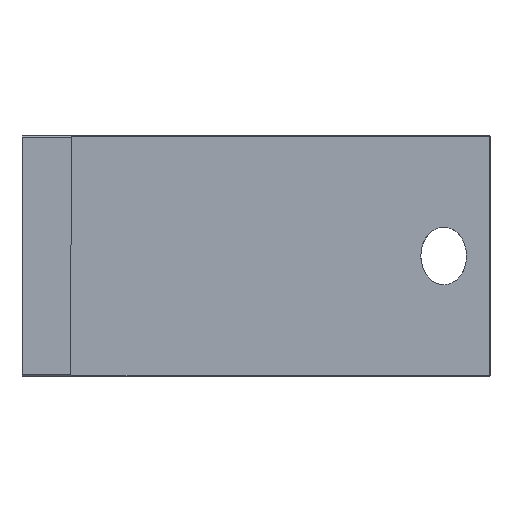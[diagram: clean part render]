
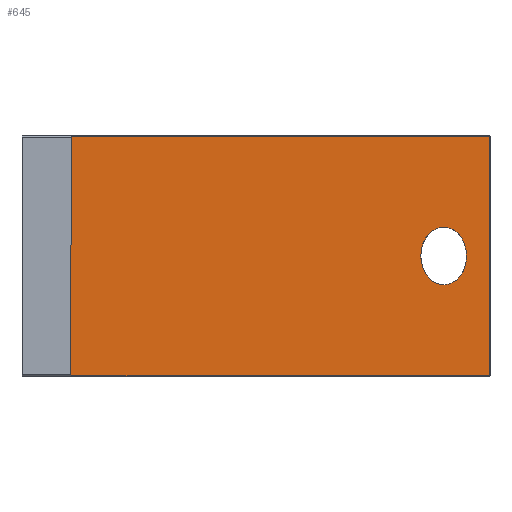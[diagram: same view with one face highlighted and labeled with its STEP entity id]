
A CAD part, left-side view. The second image highlights one B-rep face of the part: STEP entity #645.
In plain terms, the highlighted planar face has unit normal (-1, 0, 0).
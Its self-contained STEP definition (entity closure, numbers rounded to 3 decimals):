
#16=FACE_BOUND('',#121,.T.);
#17=ELLIPSE('',#684,1.104,0.873);
#18=ELLIPSE('',#685,1.104,0.873);
#49=PLANE('',#711);
#84=FACE_OUTER_BOUND('',#120,.T.);
#120=EDGE_LOOP('',(#591,#592,#593,#594));
#121=EDGE_LOOP('',(#595,#596));
#178=LINE('',#1037,#255);
#191=LINE('',#1061,#268);
#194=LINE('',#1067,#271);
#199=LINE('',#1078,#276);
#255=VECTOR('',#830,10.);
#268=VECTOR('',#855,10.);
#271=VECTOR('',#862,10.);
#276=VECTOR('',#877,1000.);
#310=VERTEX_POINT('',#967);
#311=VERTEX_POINT('',#968);
#332=VERTEX_POINT('',#1029);
#334=VERTEX_POINT('',#1035);
#338=VERTEX_POINT('',#1054);
#340=VERTEX_POINT('',#1065);
#373=EDGE_CURVE('',#310,#311,#17,.T.);
#374=EDGE_CURVE('',#311,#310,#18,.T.);
#408=EDGE_CURVE('',#332,#334,#178,.T.);
#421=EDGE_CURVE('',#338,#332,#191,.T.);
#424=EDGE_CURVE('',#340,#338,#194,.T.);
#429=EDGE_CURVE('',#340,#334,#199,.T.);
#591=ORIENTED_EDGE('',*,*,#424,.F.);
#592=ORIENTED_EDGE('',*,*,#429,.T.);
#593=ORIENTED_EDGE('',*,*,#408,.F.);
#594=ORIENTED_EDGE('',*,*,#421,.F.);
#595=ORIENTED_EDGE('',*,*,#373,.T.);
#596=ORIENTED_EDGE('',*,*,#374,.T.);
#645=ADVANCED_FACE('',(#84,#16),#49,.F.);
#684=AXIS2_PLACEMENT_3D('',#969,#771,#772);
#685=AXIS2_PLACEMENT_3D('',#970,#773,#774);
#711=AXIS2_PLACEMENT_3D('',#1079,#878,#879);
#771=DIRECTION('center_axis',(1.,0.,0.));
#772=DIRECTION('ref_axis',(0.,0.,1.));
#773=DIRECTION('center_axis',(1.,0.,0.));
#774=DIRECTION('ref_axis',(0.,0.,1.));
#830=DIRECTION('',(0.,1.,0.));
#855=DIRECTION('',(0.,0.,-1.));
#862=DIRECTION('',(0.,-1.,0.));
#877=DIRECTION('',(0.,0.001,-1.));
#878=DIRECTION('center_axis',(1.,0.,0.));
#879=DIRECTION('ref_axis',(0.,1.,0.));
#967=CARTESIAN_POINT('',(-14.424,-19.812,5.704));
#968=CARTESIAN_POINT('',(-14.424,-19.812,3.496));
#969=CARTESIAN_POINT('Origin',(-14.424,-19.812,4.6));
#970=CARTESIAN_POINT('Origin',(-14.424,-19.812,4.6));
#1029=CARTESIAN_POINT('',(-14.424,-21.577,0.01));
#1035=CARTESIAN_POINT('',(-14.424,-5.53,0.01));
#1037=CARTESIAN_POINT('',(-14.424,-10.794,0.01));
#1054=CARTESIAN_POINT('',(-14.424,-21.577,9.19));
#1061=CARTESIAN_POINT('',(-14.424,-21.577,9.2));
#1065=CARTESIAN_POINT('',(-14.424,-5.538,9.19));
#1067=CARTESIAN_POINT('',(-14.424,-10.794,9.19));
#1078=CARTESIAN_POINT('',(-14.424,-5.538,9.2));
#1079=CARTESIAN_POINT('Origin',(-14.424,-21.587,9.2));
